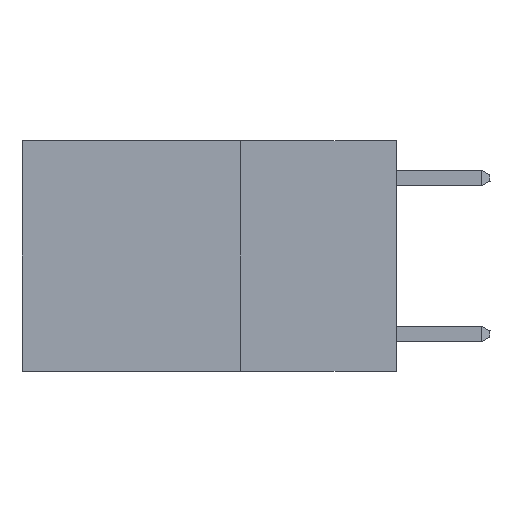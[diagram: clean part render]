
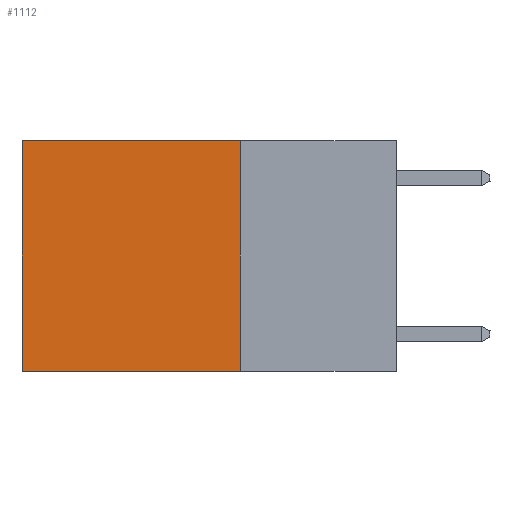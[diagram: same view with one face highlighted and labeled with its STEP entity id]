
A CAD part, left-side view. The second image highlights one B-rep face of the part: STEP entity #1112.
In plain terms, the highlighted planar face has unit normal (-1, 0, 0).
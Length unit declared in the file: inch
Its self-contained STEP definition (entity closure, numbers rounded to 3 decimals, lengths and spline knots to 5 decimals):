
#878 = CARTESIAN_POINT ( 'NONE',  ( 0.2625, 0.6, 0. ) ) ;
#1112 = ADVANCED_FACE ( 'NONE', ( #2472 ), #9765, .F. ) ;
#1573 = VERTEX_POINT ( 'NONE', #12853 ) ;
#1858 = LINE ( 'NONE', #878, #9299 ) ;
#2341 = VECTOR ( 'NONE', #10698, 39.37008 ) ;
#2418 = ORIENTED_EDGE ( 'NONE', *, *, #4091, .F. ) ;
#2472 = FACE_OUTER_BOUND ( 'NONE', #12670, .T. ) ;
#2619 = VERTEX_POINT ( 'NONE', #9999 ) ;
#2736 = DIRECTION ( 'NONE',  ( 0., 0., -1. ) ) ;
#3438 = CARTESIAN_POINT ( 'NONE',  ( 0.2625, 0.25, 0. ) ) ;
#3467 = EDGE_CURVE ( 'NONE', #2619, #10446, #9259, .T. ) ;
#3578 = DIRECTION ( 'NONE',  ( 1., 0., 0. ) ) ;
#3766 = AXIS2_PLACEMENT_3D ( 'NONE', #3438, #3578, #11097 ) ;
#4034 = CARTESIAN_POINT ( 'NONE',  ( 0.2625, 0.25, 0. ) ) ;
#4091 = EDGE_CURVE ( 'NONE', #10586, #1573, #6301, .T. ) ;
#4214 = CARTESIAN_POINT ( 'NONE',  ( 0.2625, 0.25, -0.37 ) ) ;
#6301 = LINE ( 'NONE', #4214, #12007 ) ;
#6935 = EDGE_CURVE ( 'NONE', #2619, #10586, #9454, .T. ) ;
#7397 = VECTOR ( 'NONE', #11139, 39.37008 ) ;
#7685 = EDGE_CURVE ( 'NONE', #10446, #1573, #1858, .T. ) ;
#8485 = CARTESIAN_POINT ( 'NONE',  ( 0.2625, 0.25, 0. ) ) ;
#8678 = ORIENTED_EDGE ( 'NONE', *, *, #6935, .F. ) ;
#9259 = LINE ( 'NONE', #4034, #7397 ) ;
#9299 = VECTOR ( 'NONE', #2736, 39.37008 ) ;
#9454 = LINE ( 'NONE', #8485, #2341 ) ;
#9765 = PLANE ( 'NONE',  #3766 ) ;
#9999 = CARTESIAN_POINT ( 'NONE',  ( 0.2625, 0.25, 0. ) ) ;
#10446 = VERTEX_POINT ( 'NONE', #11336 ) ;
#10586 = VERTEX_POINT ( 'NONE', #11662 ) ;
#10698 = DIRECTION ( 'NONE',  ( 0., 0., -1. ) ) ;
#11097 = DIRECTION ( 'NONE',  ( 0., 0., -1. ) ) ;
#11139 = DIRECTION ( 'NONE',  ( 0., 1., 0. ) ) ;
#11336 = CARTESIAN_POINT ( 'NONE',  ( 0.2625, 0.6, 0. ) ) ;
#11343 = ORIENTED_EDGE ( 'NONE', *, *, #7685, .T. ) ;
#11662 = CARTESIAN_POINT ( 'NONE',  ( 0.2625, 0.25, -0.37 ) ) ;
#12007 = VECTOR ( 'NONE', #12619, 39.37008 ) ;
#12619 = DIRECTION ( 'NONE',  ( 0., 1., 0. ) ) ;
#12670 = EDGE_LOOP ( 'NONE', ( #11343, #2418, #8678, #13270 ) ) ;
#12853 = CARTESIAN_POINT ( 'NONE',  ( 0.2625, 0.6, -0.37 ) ) ;
#13270 = ORIENTED_EDGE ( 'NONE', *, *, #3467, .T. ) ;
